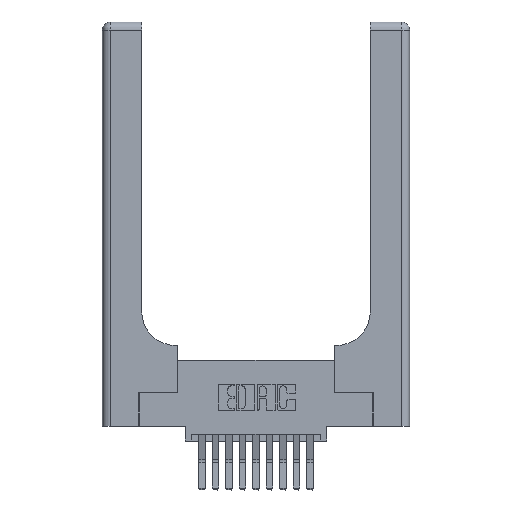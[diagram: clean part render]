
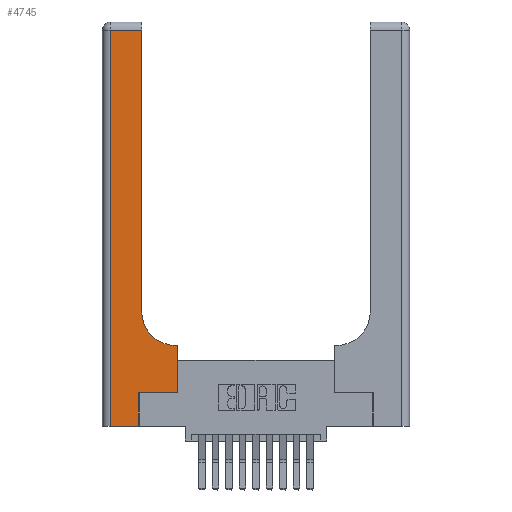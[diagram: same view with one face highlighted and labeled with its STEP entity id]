
A CAD part, top view. The second image highlights one B-rep face of the part: STEP entity #4745.
In plain terms, the highlighted planar face has unit normal (0, 0, 1).
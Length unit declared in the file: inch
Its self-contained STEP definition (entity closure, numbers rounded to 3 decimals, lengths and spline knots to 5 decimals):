
#473 = ORIENTED_EDGE ( 'NONE', *, *, #12901, .T. ) ;
#629 = DIRECTION ( 'NONE',  ( 0., 1., 0. ) ) ;
#832 = LINE ( 'NONE', #7906, #14533 ) ;
#1006 = DIRECTION ( 'NONE',  ( 0., 1., 0. ) ) ;
#1064 = EDGE_CURVE ( 'NONE', #16322, #2865, #8135, .T. ) ;
#1149 = VECTOR ( 'NONE', #1006, 39.37008 ) ;
#1308 = LINE ( 'NONE', #1742, #16437 ) ;
#1594 = LINE ( 'NONE', #1864, #11228 ) ;
#1742 = CARTESIAN_POINT ( 'NONE',  ( 0., 2.94, 0.37 ) ) ;
#1864 = CARTESIAN_POINT ( 'NONE',  ( 0.2915, 0.6, 0.37 ) ) ;
#2466 = CARTESIAN_POINT ( 'NONE',  ( 0.269, 0., 0.37 ) ) ;
#2672 = ORIENTED_EDGE ( 'NONE', *, *, #11841, .T. ) ;
#2865 = VERTEX_POINT ( 'NONE', #12590 ) ;
#2928 = EDGE_CURVE ( 'NONE', #5676, #5582, #1308, .T. ) ;
#3341 = LINE ( 'NONE', #13486, #6464 ) ;
#3795 = VECTOR ( 'NONE', #11510, 39.37008 ) ;
#3821 = EDGE_CURVE ( 'NONE', #2865, #13029, #15457, .T. ) ;
#3984 = VERTEX_POINT ( 'NONE', #11050 ) ;
#4029 = EDGE_CURVE ( 'NONE', #13029, #3984, #6268, .T. ) ;
#4183 = CARTESIAN_POINT ( 'NONE',  ( 0.5585, 0.25, 0.37 ) ) ;
#4525 = CARTESIAN_POINT ( 'NONE',  ( 0.2915, 0.85, 0.37 ) ) ;
#4745 = ADVANCED_FACE ( 'NONE', ( #10782 ), #15832, .F. ) ;
#4930 = CARTESIAN_POINT ( 'NONE',  ( 0.269, 0.25, 0.37 ) ) ;
#5322 = DIRECTION ( 'NONE',  ( 0., 0., -1. ) ) ;
#5582 = VERTEX_POINT ( 'NONE', #5912 ) ;
#5676 = VERTEX_POINT ( 'NONE', #7585 ) ;
#5912 = CARTESIAN_POINT ( 'NONE',  ( 0.06, 2.94, 0.37 ) ) ;
#6132 = ORIENTED_EDGE ( 'NONE', *, *, #2928, .T. ) ;
#6268 = LINE ( 'NONE', #8505, #6466 ) ;
#6373 = AXIS2_PLACEMENT_3D ( 'NONE', #13242, #5322, #15597 ) ;
#6464 = VECTOR ( 'NONE', #12361, 39.37008 ) ;
#6466 = VECTOR ( 'NONE', #629, 39.37008 ) ;
#7419 = ORIENTED_EDGE ( 'NONE', *, *, #3821, .T. ) ;
#7585 = CARTESIAN_POINT ( 'NONE',  ( 0.2915, 2.94, 0.37 ) ) ;
#7626 = EDGE_CURVE ( 'NONE', #5582, #8990, #832, .T. ) ;
#7761 = CARTESIAN_POINT ( 'NONE',  ( 0., 0., 0.37 ) ) ;
#7906 = CARTESIAN_POINT ( 'NONE',  ( 0.06, 3., 0.37 ) ) ;
#7990 = VERTEX_POINT ( 'NONE', #4525 ) ;
#8135 = LINE ( 'NONE', #12718, #1149 ) ;
#8196 = VERTEX_POINT ( 'NONE', #15386 ) ;
#8505 = CARTESIAN_POINT ( 'NONE',  ( 0.5585, 0.25, 0.37 ) ) ;
#8635 = AXIS2_PLACEMENT_3D ( 'NONE', #14323, #11810, #14436 ) ;
#8710 = EDGE_CURVE ( 'NONE', #8990, #16322, #9046, .T. ) ;
#8990 = VERTEX_POINT ( 'NONE', #16101 ) ;
#9046 = LINE ( 'NONE', #7761, #12858 ) ;
#9119 = EDGE_CURVE ( 'NONE', #3984, #8196, #1594, .T. ) ;
#9660 = ORIENTED_EDGE ( 'NONE', *, *, #4029, .T. ) ;
#10162 = CIRCLE ( 'NONE', #8635, 0.25 ) ;
#10293 = ORIENTED_EDGE ( 'NONE', *, *, #8710, .T. ) ;
#10782 = FACE_OUTER_BOUND ( 'NONE', #14635, .T. ) ;
#11050 = CARTESIAN_POINT ( 'NONE',  ( 0.5585, 0.6, 0.37 ) ) ;
#11228 = VECTOR ( 'NONE', #12389, 39.37008 ) ;
#11510 = DIRECTION ( 'NONE',  ( 1., 0., 0. ) ) ;
#11616 = DIRECTION ( 'NONE',  ( 1., 0., 0. ) ) ;
#11810 = DIRECTION ( 'NONE',  ( 0., 0., -1. ) ) ;
#11841 = EDGE_CURVE ( 'NONE', #7990, #5676, #3341, .T. ) ;
#12361 = DIRECTION ( 'NONE',  ( 0., 1., 0. ) ) ;
#12389 = DIRECTION ( 'NONE',  ( -1., 0., 0. ) ) ;
#12565 = ORIENTED_EDGE ( 'NONE', *, *, #7626, .T. ) ;
#12590 = CARTESIAN_POINT ( 'NONE',  ( 0.269, 0.25, 0.37 ) ) ;
#12718 = CARTESIAN_POINT ( 'NONE',  ( 0.269, 0., 0.37 ) ) ;
#12858 = VECTOR ( 'NONE', #11616, 39.37008 ) ;
#12901 = EDGE_CURVE ( 'NONE', #8196, #7990, #10162, .T. ) ;
#13029 = VERTEX_POINT ( 'NONE', #4183 ) ;
#13234 = ORIENTED_EDGE ( 'NONE', *, *, #9119, .T. ) ;
#13242 = CARTESIAN_POINT ( 'NONE',  ( 0., 3., 0.37 ) ) ;
#13486 = CARTESIAN_POINT ( 'NONE',  ( 0.2915, 3., 0.37 ) ) ;
#14323 = CARTESIAN_POINT ( 'NONE',  ( 0.5415, 0.85, 0.37 ) ) ;
#14324 = DIRECTION ( 'NONE',  ( 0., -1., 0. ) ) ;
#14436 = DIRECTION ( 'NONE',  ( 1., 0., 0. ) ) ;
#14533 = VECTOR ( 'NONE', #14324, 39.37008 ) ;
#14635 = EDGE_LOOP ( 'NONE', ( #2672, #6132, #12565, #10293, #16674, #7419, #9660, #13234, #473 ) ) ;
#14714 = DIRECTION ( 'NONE',  ( -1., 0., 0. ) ) ;
#15386 = CARTESIAN_POINT ( 'NONE',  ( 0.5415, 0.6, 0.37 ) ) ;
#15457 = LINE ( 'NONE', #4930, #3795 ) ;
#15597 = DIRECTION ( 'NONE',  ( -1., 0., 0. ) ) ;
#15832 = PLANE ( 'NONE',  #6373 ) ;
#16101 = CARTESIAN_POINT ( 'NONE',  ( 0.06, 0., 0.37 ) ) ;
#16322 = VERTEX_POINT ( 'NONE', #2466 ) ;
#16437 = VECTOR ( 'NONE', #14714, 39.37008 ) ;
#16674 = ORIENTED_EDGE ( 'NONE', *, *, #1064, .T. ) ;
